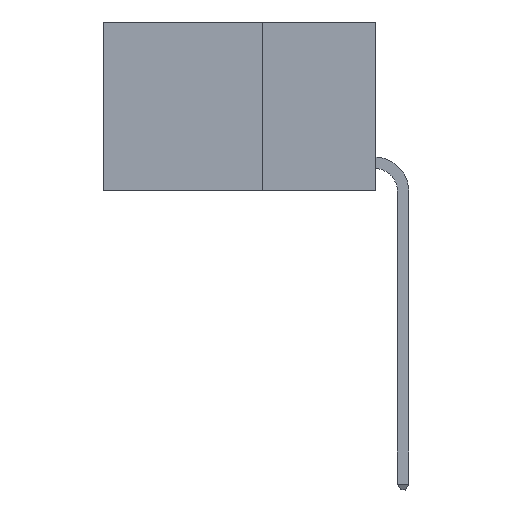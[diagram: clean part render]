
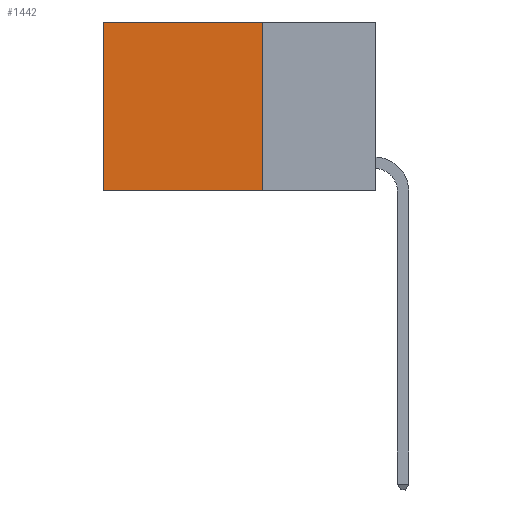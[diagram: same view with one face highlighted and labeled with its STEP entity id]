
A CAD part, left-side view. The second image highlights one B-rep face of the part: STEP entity #1442.
In plain terms, the highlighted planar face has unit normal (-1, 0, 0).
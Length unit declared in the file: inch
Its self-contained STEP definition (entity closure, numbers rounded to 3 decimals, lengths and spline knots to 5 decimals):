
#126 = VERTEX_POINT ( 'NONE', #2601 ) ;
#515 = DIRECTION ( 'NONE',  ( 0., 0., -1. ) ) ;
#1387 = CARTESIAN_POINT ( 'NONE',  ( 0.2625, 0.6, -0.37 ) ) ;
#1442 = ADVANCED_FACE ( 'NONE', ( #14546 ), #7801, .F. ) ;
#2601 = CARTESIAN_POINT ( 'NONE',  ( 0.2625, 0.6, 0. ) ) ;
#3917 = CARTESIAN_POINT ( 'NONE',  ( 0.2625, 0.6, 0. ) ) ;
#3991 = CARTESIAN_POINT ( 'NONE',  ( 0.2625, 0.25, 0. ) ) ;
#4282 = LINE ( 'NONE', #3917, #10712 ) ;
#4658 = VERTEX_POINT ( 'NONE', #1387 ) ;
#5529 = LINE ( 'NONE', #17882, #8701 ) ;
#5633 = LINE ( 'NONE', #9178, #8811 ) ;
#7072 = ORIENTED_EDGE ( 'NONE', *, *, #15890, .F. ) ;
#7632 = ORIENTED_EDGE ( 'NONE', *, *, #8041, .T. ) ;
#7801 = PLANE ( 'NONE',  #9280 ) ;
#7902 = ORIENTED_EDGE ( 'NONE', *, *, #12148, .F. ) ;
#8041 = EDGE_CURVE ( 'NONE', #12587, #126, #10093, .T. ) ;
#8701 = VECTOR ( 'NONE', #9759, 39.37008 ) ;
#8811 = VECTOR ( 'NONE', #17372, 39.37008 ) ;
#9159 = DIRECTION ( 'NONE',  ( 1., 0., 0. ) ) ;
#9178 = CARTESIAN_POINT ( 'NONE',  ( 0.2625, 0.25, -0.37 ) ) ;
#9280 = AXIS2_PLACEMENT_3D ( 'NONE', #17305, #9159, #515 ) ;
#9759 = DIRECTION ( 'NONE',  ( 0., 0., -1. ) ) ;
#10093 = LINE ( 'NONE', #3991, #13350 ) ;
#10593 = ORIENTED_EDGE ( 'NONE', *, *, #15993, .T. ) ;
#10600 = CARTESIAN_POINT ( 'NONE',  ( 0.2625, 0.25, 0. ) ) ;
#10712 = VECTOR ( 'NONE', #14940, 39.37008 ) ;
#12148 = EDGE_CURVE ( 'NONE', #12587, #13019, #5529, .T. ) ;
#12250 = DIRECTION ( 'NONE',  ( 0., 1., 0. ) ) ;
#12587 = VERTEX_POINT ( 'NONE', #10600 ) ;
#13019 = VERTEX_POINT ( 'NONE', #14109 ) ;
#13350 = VECTOR ( 'NONE', #12250, 39.37008 ) ;
#14109 = CARTESIAN_POINT ( 'NONE',  ( 0.2625, 0.25, -0.37 ) ) ;
#14546 = FACE_OUTER_BOUND ( 'NONE', #17949, .T. ) ;
#14940 = DIRECTION ( 'NONE',  ( 0., 0., -1. ) ) ;
#15890 = EDGE_CURVE ( 'NONE', #13019, #4658, #5633, .T. ) ;
#15993 = EDGE_CURVE ( 'NONE', #126, #4658, #4282, .T. ) ;
#17305 = CARTESIAN_POINT ( 'NONE',  ( 0.2625, 0.25, 0. ) ) ;
#17372 = DIRECTION ( 'NONE',  ( 0., 1., 0. ) ) ;
#17882 = CARTESIAN_POINT ( 'NONE',  ( 0.2625, 0.25, 0. ) ) ;
#17949 = EDGE_LOOP ( 'NONE', ( #10593, #7072, #7902, #7632 ) ) ;
